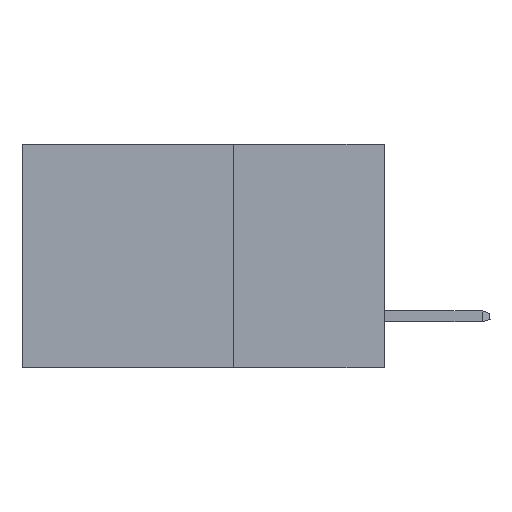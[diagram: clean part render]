
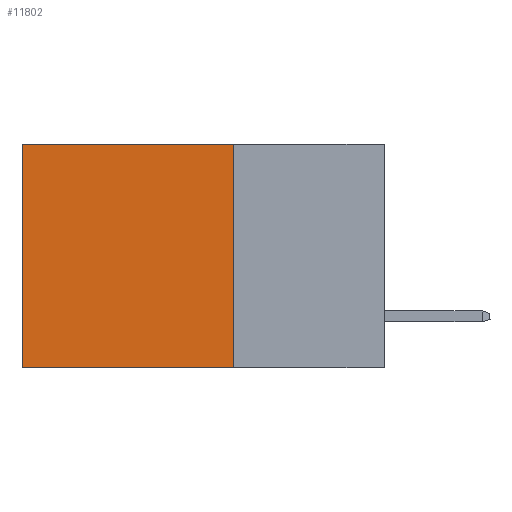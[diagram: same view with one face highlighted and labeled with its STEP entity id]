
A CAD part, left-side view. The second image highlights one B-rep face of the part: STEP entity #11802.
In plain terms, the highlighted planar face has unit normal (-1, 0, 0).
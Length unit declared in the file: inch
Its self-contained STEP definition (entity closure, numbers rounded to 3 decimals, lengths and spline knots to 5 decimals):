
#1190 = LINE ( 'NONE', #22587, #24691 ) ;
#1338 = DIRECTION ( 'NONE',  ( 0., 0., -1. ) ) ;
#1391 = LINE ( 'NONE', #13626, #17481 ) ;
#1905 = LINE ( 'NONE', #13260, #7266 ) ;
#4032 = EDGE_CURVE ( 'NONE', #21811, #20380, #1391, .T. ) ;
#5072 = PLANE ( 'NONE',  #5771 ) ;
#5771 = AXIS2_PLACEMENT_3D ( 'NONE', #27689, #9677, #25537 ) ;
#6519 = DIRECTION ( 'NONE',  ( 0., 0., -1. ) ) ;
#7063 = CARTESIAN_POINT ( 'NONE',  ( 0.298, 0.25, -0.37 ) ) ;
#7266 = VECTOR ( 'NONE', #6519, 39.37008 ) ;
#8412 = ORIENTED_EDGE ( 'NONE', *, *, #4032, .F. ) ;
#9317 = DIRECTION ( 'NONE',  ( 0., 1., 0. ) ) ;
#9677 = DIRECTION ( 'NONE',  ( 1., 0., 0. ) ) ;
#10201 = CARTESIAN_POINT ( 'NONE',  ( 0.298, 0.6, -0.37 ) ) ;
#10835 = LINE ( 'NONE', #23017, #16215 ) ;
#11802 = ADVANCED_FACE ( 'NONE', ( #23054 ), #5072, .F. ) ;
#13260 = CARTESIAN_POINT ( 'NONE',  ( 0.298, 0.6, 0. ) ) ;
#13626 = CARTESIAN_POINT ( 'NONE',  ( 0.298, 0.25, 0. ) ) ;
#13713 = CARTESIAN_POINT ( 'NONE',  ( 0.298, 0.25, 0. ) ) ;
#15311 = ORIENTED_EDGE ( 'NONE', *, *, #25069, .T. ) ;
#16215 = VECTOR ( 'NONE', #9317, 39.37008 ) ;
#16801 = EDGE_LOOP ( 'NONE', ( #23457, #22470, #8412, #15311 ) ) ;
#17481 = VECTOR ( 'NONE', #1338, 39.37008 ) ;
#17714 = VERTEX_POINT ( 'NONE', #20041 ) ;
#20041 = CARTESIAN_POINT ( 'NONE',  ( 0.298, 0.6, 0. ) ) ;
#20085 = VERTEX_POINT ( 'NONE', #10201 ) ;
#20380 = VERTEX_POINT ( 'NONE', #7063 ) ;
#21811 = VERTEX_POINT ( 'NONE', #13713 ) ;
#22470 = ORIENTED_EDGE ( 'NONE', *, *, #23706, .F. ) ;
#22587 = CARTESIAN_POINT ( 'NONE',  ( 0.298, 0.25, -0.37 ) ) ;
#23017 = CARTESIAN_POINT ( 'NONE',  ( 0.298, 0.25, 0. ) ) ;
#23054 = FACE_OUTER_BOUND ( 'NONE', #16801, .T. ) ;
#23457 = ORIENTED_EDGE ( 'NONE', *, *, #24328, .T. ) ;
#23706 = EDGE_CURVE ( 'NONE', #20380, #20085, #1190, .T. ) ;
#24328 = EDGE_CURVE ( 'NONE', #17714, #20085, #1905, .T. ) ;
#24691 = VECTOR ( 'NONE', #24859, 39.37008 ) ;
#24859 = DIRECTION ( 'NONE',  ( 0., 1., 0. ) ) ;
#25069 = EDGE_CURVE ( 'NONE', #21811, #17714, #10835, .T. ) ;
#25537 = DIRECTION ( 'NONE',  ( 0., 0., -1. ) ) ;
#27689 = CARTESIAN_POINT ( 'NONE',  ( 0.298, 0.25, 0. ) ) ;
